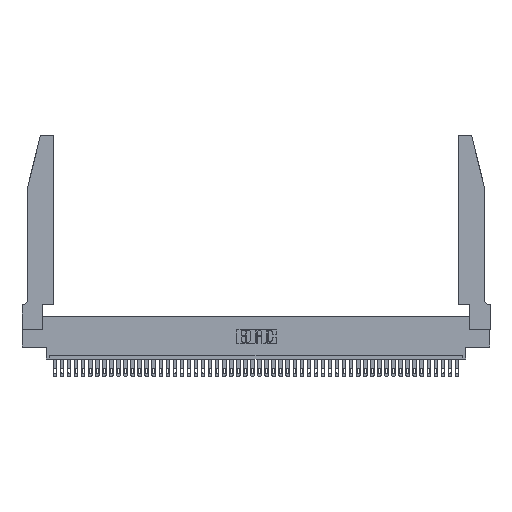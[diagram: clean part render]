
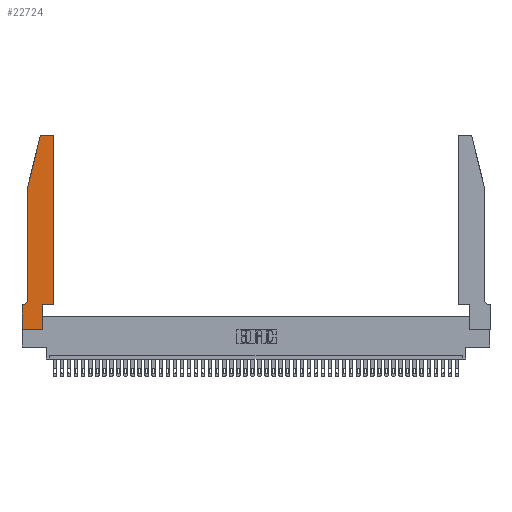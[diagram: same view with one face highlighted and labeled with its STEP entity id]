
A CAD part, top view. The second image highlights one B-rep face of the part: STEP entity #22724.
In plain terms, the highlighted planar face has unit normal (0, 0, 1).
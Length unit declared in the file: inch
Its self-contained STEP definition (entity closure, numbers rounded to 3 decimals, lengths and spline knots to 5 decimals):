
#184 = EDGE_LOOP ( 'NONE', ( #34945, #1369, #925, #11586, #34412, #4068, #10953, #42157, #46232, #38203, #37088, #36765 ) ) ;
#226 = EDGE_CURVE ( 'NONE', #10311, #35224, #19973, .T. ) ;
#798 = CARTESIAN_POINT ( 'NONE',  ( 0.0755, 2., 0.37 ) ) ;
#925 = ORIENTED_EDGE ( 'NONE', *, *, #28963, .T. ) ;
#1369 = ORIENTED_EDGE ( 'NONE', *, *, #29896, .T. ) ;
#1681 = CIRCLE ( 'NONE', #8347, 0.07 ) ;
#2275 = EDGE_CURVE ( 'NONE', #10880, #37542, #32080, .T. ) ;
#2725 = CARTESIAN_POINT ( 'NONE',  ( 0.4505, 0.35, 0.37 ) ) ;
#2907 = LINE ( 'NONE', #45630, #39698 ) ;
#4068 = ORIENTED_EDGE ( 'NONE', *, *, #32752, .T. ) ;
#4339 = CARTESIAN_POINT ( 'NONE',  ( 0.0055, 0.42, 0.37 ) ) ;
#6360 = CARTESIAN_POINT ( 'NONE',  ( 0.4205, 2.75, 0.37 ) ) ;
#7395 = AXIS2_PLACEMENT_3D ( 'NONE', #12634, #45473, #24105 ) ;
#8347 = AXIS2_PLACEMENT_3D ( 'NONE', #4339, #22467, #29358 ) ;
#9822 = VECTOR ( 'NONE', #27652, 39.37008 ) ;
#9861 = CARTESIAN_POINT ( 'NONE',  ( 0., 0.35, 0.37 ) ) ;
#10042 = CARTESIAN_POINT ( 'NONE',  ( 0.284, 2.75, 0.37 ) ) ;
#10311 = VERTEX_POINT ( 'NONE', #24270 ) ;
#10340 = CIRCLE ( 'NONE', #29069, 0.03 ) ;
#10618 = LINE ( 'NONE', #2725, #12248 ) ;
#10652 = CARTESIAN_POINT ( 'NONE',  ( 0., 0.35, 0.37 ) ) ;
#10809 = EDGE_CURVE ( 'NONE', #13990, #12014, #24931, .T. ) ;
#10880 = VERTEX_POINT ( 'NONE', #6360 ) ;
#10953 = ORIENTED_EDGE ( 'NONE', *, *, #19166, .T. ) ;
#11141 = CARTESIAN_POINT ( 'NONE',  ( 0., 0., 0.37 ) ) ;
#11160 = AXIS2_PLACEMENT_3D ( 'NONE', #9861, #34858, #13436 ) ;
#11352 = VERTEX_POINT ( 'NONE', #22670 ) ;
#11586 = ORIENTED_EDGE ( 'NONE', *, *, #10809, .T. ) ;
#12014 = VERTEX_POINT ( 'NONE', #40302 ) ;
#12248 = VECTOR ( 'NONE', #27756, 39.37008 ) ;
#12463 = VECTOR ( 'NONE', #31939, 39.37008 ) ;
#12634 = CARTESIAN_POINT ( 'NONE',  ( 0.4205, 2.72, 0.37 ) ) ;
#13436 = DIRECTION ( 'NONE',  ( 1., 0., 0. ) ) ;
#13990 = VERTEX_POINT ( 'NONE', #798 ) ;
#14334 = VERTEX_POINT ( 'NONE', #19372 ) ;
#14970 = VERTEX_POINT ( 'NONE', #41421 ) ;
#15138 = EDGE_CURVE ( 'NONE', #40670, #10880, #33681, .T. ) ;
#15277 = VECTOR ( 'NONE', #34169, 39.37008 ) ;
#16783 = EDGE_CURVE ( 'NONE', #14334, #40670, #10618, .T. ) ;
#17328 = DIRECTION ( 'NONE',  ( -1., 0., 0. ) ) ;
#18263 = VECTOR ( 'NONE', #25865, 39.37008 ) ;
#19166 = EDGE_CURVE ( 'NONE', #21214, #10311, #2907, .T. ) ;
#19196 = VECTOR ( 'NONE', #31155, 39.37008 ) ;
#19249 = EDGE_CURVE ( 'NONE', #12014, #14970, #1681, .T. ) ;
#19372 = CARTESIAN_POINT ( 'NONE',  ( 0.4505, 0.35, 0.37 ) ) ;
#19410 = CARTESIAN_POINT ( 'NONE',  ( 0.284, 2.72, 0.37 ) ) ;
#19715 = VECTOR ( 'NONE', #23810, 39.37008 ) ;
#19973 = LINE ( 'NONE', #11141, #18263 ) ;
#21214 = VERTEX_POINT ( 'NONE', #10652 ) ;
#22467 = DIRECTION ( 'NONE',  ( 0., 0., -1. ) ) ;
#22670 = CARTESIAN_POINT ( 'NONE',  ( 0.2865, 0.35, 0.37 ) ) ;
#22724 = ADVANCED_FACE ( 'NONE', ( #38601 ), #27746, .T. ) ;
#23755 = CARTESIAN_POINT ( 'NONE',  ( 0.0755, 2., 0.37 ) ) ;
#23810 = DIRECTION ( 'NONE',  ( 0., 1., 0. ) ) ;
#24105 = DIRECTION ( 'NONE',  ( 1., 0., 0. ) ) ;
#24270 = CARTESIAN_POINT ( 'NONE',  ( 0., 0., 0.37 ) ) ;
#24931 = LINE ( 'NONE', #23755, #15277 ) ;
#24992 = VERTEX_POINT ( 'NONE', #29385 ) ;
#25865 = DIRECTION ( 'NONE',  ( 1., 0., 0. ) ) ;
#26748 = CARTESIAN_POINT ( 'NONE',  ( 0.2605, 2.75, 0.37 ) ) ;
#27652 = DIRECTION ( 'NONE',  ( -0.239, -0.971, 0. ) ) ;
#27746 = PLANE ( 'NONE',  #11160 ) ;
#27756 = DIRECTION ( 'NONE',  ( 0., 1., 0. ) ) ;
#28208 = LINE ( 'NONE', #35503, #12463 ) ;
#28282 = CARTESIAN_POINT ( 'NONE',  ( 0.2865, 0., 0.37 ) ) ;
#28963 = EDGE_CURVE ( 'NONE', #24992, #13990, #42237, .T. ) ;
#29069 = AXIS2_PLACEMENT_3D ( 'NONE', #19410, #35622, #34839 ) ;
#29358 = DIRECTION ( 'NONE',  ( -1., 0., 0. ) ) ;
#29385 = CARTESIAN_POINT ( 'NONE',  ( 0.25487, 2.72718, 0.37 ) ) ;
#29896 = EDGE_CURVE ( 'NONE', #37542, #24992, #10340, .T. ) ;
#30719 = DIRECTION ( 'NONE',  ( 0., -1., 0. ) ) ;
#31155 = DIRECTION ( 'NONE',  ( -1., 0., 0. ) ) ;
#31939 = DIRECTION ( 'NONE',  ( 1., 0., 0. ) ) ;
#32080 = LINE ( 'NONE', #26748, #19196 ) ;
#32115 = EDGE_CURVE ( 'NONE', #35224, #11352, #34744, .T. ) ;
#32752 = EDGE_CURVE ( 'NONE', #14970, #21214, #35249, .T. ) ;
#33681 = CIRCLE ( 'NONE', #7395, 0.03 ) ;
#34169 = DIRECTION ( 'NONE',  ( 0., -1., 0. ) ) ;
#34412 = ORIENTED_EDGE ( 'NONE', *, *, #19249, .T. ) ;
#34435 = CARTESIAN_POINT ( 'NONE',  ( 0.0755, 2., 0.37 ) ) ;
#34744 = LINE ( 'NONE', #38431, #19715 ) ;
#34839 = DIRECTION ( 'NONE',  ( 1., 0., 0. ) ) ;
#34858 = DIRECTION ( 'NONE',  ( 0., 0., 1. ) ) ;
#34945 = ORIENTED_EDGE ( 'NONE', *, *, #2275, .T. ) ;
#35224 = VERTEX_POINT ( 'NONE', #28282 ) ;
#35249 = LINE ( 'NONE', #38702, #36326 ) ;
#35503 = CARTESIAN_POINT ( 'NONE',  ( 0.4505, 0.35, 0.37 ) ) ;
#35622 = DIRECTION ( 'NONE',  ( 0., 0., 1. ) ) ;
#35693 = CARTESIAN_POINT ( 'NONE',  ( 0.4505, 2.72, 0.37 ) ) ;
#36326 = VECTOR ( 'NONE', #17328, 39.37008 ) ;
#36765 = ORIENTED_EDGE ( 'NONE', *, *, #15138, .T. ) ;
#37088 = ORIENTED_EDGE ( 'NONE', *, *, #16783, .T. ) ;
#37541 = EDGE_CURVE ( 'NONE', #11352, #14334, #28208, .T. ) ;
#37542 = VERTEX_POINT ( 'NONE', #10042 ) ;
#38203 = ORIENTED_EDGE ( 'NONE', *, *, #37541, .T. ) ;
#38431 = CARTESIAN_POINT ( 'NONE',  ( 0.2865, 0.35, 0.37 ) ) ;
#38601 = FACE_OUTER_BOUND ( 'NONE', #184, .T. ) ;
#38702 = CARTESIAN_POINT ( 'NONE',  ( 0.0755, 0.35, 0.37 ) ) ;
#39698 = VECTOR ( 'NONE', #30719, 39.37008 ) ;
#40302 = CARTESIAN_POINT ( 'NONE',  ( 0.0755, 0.42, 0.37 ) ) ;
#40670 = VERTEX_POINT ( 'NONE', #35693 ) ;
#41421 = CARTESIAN_POINT ( 'NONE',  ( 0.0055, 0.35, 0.37 ) ) ;
#42157 = ORIENTED_EDGE ( 'NONE', *, *, #226, .T. ) ;
#42237 = LINE ( 'NONE', #34435, #9822 ) ;
#45473 = DIRECTION ( 'NONE',  ( 0., 0., 1. ) ) ;
#45630 = CARTESIAN_POINT ( 'NONE',  ( 0., 0., 0.37 ) ) ;
#46232 = ORIENTED_EDGE ( 'NONE', *, *, #32115, .T. ) ;
